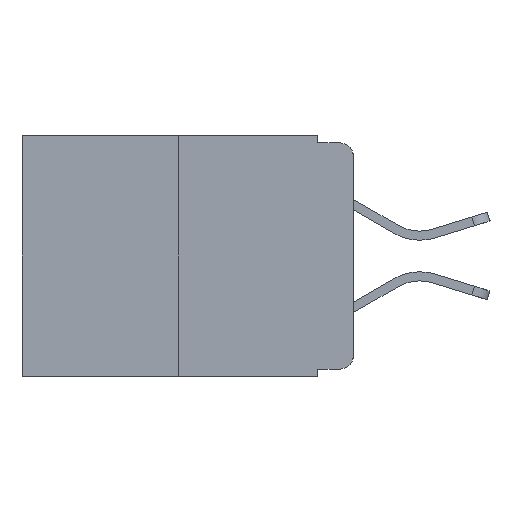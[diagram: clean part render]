
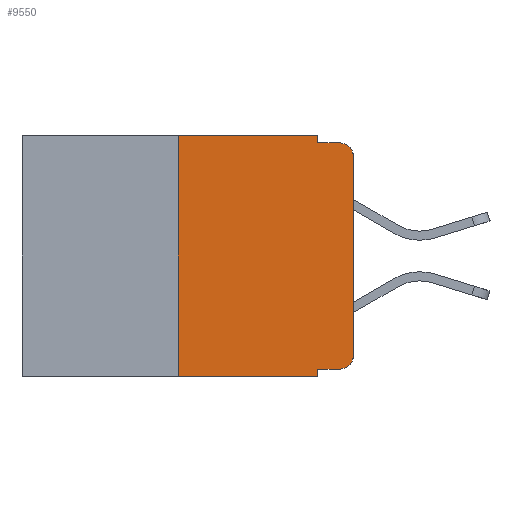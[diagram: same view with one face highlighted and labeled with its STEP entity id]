
A CAD part, left-side view. The second image highlights one B-rep face of the part: STEP entity #9550.
In plain terms, the highlighted planar face has unit normal (-1, 0, 0).
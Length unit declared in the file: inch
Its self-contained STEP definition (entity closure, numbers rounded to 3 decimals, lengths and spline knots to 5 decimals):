
#59 = VECTOR ( 'NONE', #10733, 39.37008 ) ;
#154 = AXIS2_PLACEMENT_3D ( 'NONE', #11828, #5738, #11857 ) ;
#215 = ORIENTED_EDGE ( 'NONE', *, *, #3787, .F. ) ;
#564 = ORIENTED_EDGE ( 'NONE', *, *, #3945, .F. ) ;
#913 = CARTESIAN_POINT ( 'NONE',  ( 0., 0.473, 0. ) ) ;
#932 = CIRCLE ( 'NONE', #11629, 0.02 ) ;
#991 = ORIENTED_EDGE ( 'NONE', *, *, #3729, .T. ) ;
#1109 = VECTOR ( 'NONE', #10642, 39.37008 ) ;
#1373 = VERTEX_POINT ( 'NONE', #12128 ) ;
#1569 = VERTEX_POINT ( 'NONE', #6097 ) ;
#2163 = CARTESIAN_POINT ( 'NONE',  ( 0., 0.25, 0. ) ) ;
#2320 = ORIENTED_EDGE ( 'NONE', *, *, #3783, .T. ) ;
#2646 = ORIENTED_EDGE ( 'NONE', *, *, #3926, .T. ) ;
#3071 = VECTOR ( 'NONE', #6864, 39.37008 ) ;
#3140 = CARTESIAN_POINT ( 'NONE',  ( 0., 0.051, -0.343 ) ) ;
#3144 = VECTOR ( 'NONE', #8566, 39.37008 ) ;
#3314 = LINE ( 'NONE', #11605, #8231 ) ;
#3404 = DIRECTION ( 'NONE',  ( 0., -1., 0. ) ) ;
#3415 = LINE ( 'NONE', #913, #3071 ) ;
#3512 = FACE_OUTER_BOUND ( 'NONE', #10584, .T. ) ;
#3526 = ORIENTED_EDGE ( 'NONE', *, *, #3968, .T. ) ;
#3618 = LINE ( 'NONE', #11308, #10533 ) ;
#3729 = EDGE_CURVE ( 'NONE', #11973, #4714, #6537, .T. ) ;
#3783 = EDGE_CURVE ( 'NONE', #4714, #11696, #932, .T. ) ;
#3787 = EDGE_CURVE ( 'NONE', #5689, #11696, #5661, .T. ) ;
#3902 = CARTESIAN_POINT ( 'NONE',  ( 0., 0.051, 0. ) ) ;
#3912 = EDGE_CURVE ( 'NONE', #5344, #5689, #11057, .T. ) ;
#3914 = EDGE_CURVE ( 'NONE', #1569, #8278, #3940, .T. ) ;
#3926 = EDGE_CURVE ( 'NONE', #4440, #1373, #3618, .T. ) ;
#3940 = LINE ( 'NONE', #11932, #6104 ) ;
#3945 = EDGE_CURVE ( 'NONE', #4440, #7474, #3314, .T. ) ;
#3968 = EDGE_CURVE ( 'NONE', #1373, #11973, #7937, .T. ) ;
#4101 = VECTOR ( 'NONE', #5047, 39.37008 ) ;
#4348 = DIRECTION ( 'NONE',  ( 0., 0., -1. ) ) ;
#4440 = VERTEX_POINT ( 'NONE', #9149 ) ;
#4520 = CARTESIAN_POINT ( 'NONE',  ( 0., 0.473, -0.343 ) ) ;
#4714 = VERTEX_POINT ( 'NONE', #7697 ) ;
#4834 = PLANE ( 'NONE',  #154 ) ;
#5047 = DIRECTION ( 'NONE',  ( 0., 0., 1. ) ) ;
#5276 = LINE ( 'NONE', #4520, #59 ) ;
#5344 = VERTEX_POINT ( 'NONE', #3902 ) ;
#5661 = LINE ( 'NONE', #6127, #3144 ) ;
#5689 = VERTEX_POINT ( 'NONE', #9738 ) ;
#5738 = DIRECTION ( 'NONE',  ( 1., 0., 0. ) ) ;
#5797 = CARTESIAN_POINT ( 'NONE',  ( 0., 0.02, -0.01 ) ) ;
#6089 = DIRECTION ( 'NONE',  ( 0., 0., 1. ) ) ;
#6097 = CARTESIAN_POINT ( 'NONE',  ( 0., 0.25, -0.343 ) ) ;
#6104 = VECTOR ( 'NONE', #6089, 39.37008 ) ;
#6127 = CARTESIAN_POINT ( 'NONE',  ( 0., 0.051, -0.01 ) ) ;
#6133 = AXIS2_PLACEMENT_3D ( 'NONE', #10855, #11902, #8687 ) ;
#6362 = ORIENTED_EDGE ( 'NONE', *, *, #3912, .F. ) ;
#6537 = LINE ( 'NONE', #10196, #4101 ) ;
#6864 = DIRECTION ( 'NONE',  ( 0., -1., 0. ) ) ;
#7067 = ORIENTED_EDGE ( 'NONE', *, *, #7230, .F. ) ;
#7163 = ORIENTED_EDGE ( 'NONE', *, *, #3914, .F. ) ;
#7208 = DIRECTION ( 'NONE',  ( -1., 0., 0. ) ) ;
#7230 = EDGE_CURVE ( 'NONE', #8278, #5344, #3415, .T. ) ;
#7474 = VERTEX_POINT ( 'NONE', #3140 ) ;
#7697 = CARTESIAN_POINT ( 'NONE',  ( 0., 0., -0.03 ) ) ;
#7937 = CIRCLE ( 'NONE', #6133, 0.02 ) ;
#7986 = CARTESIAN_POINT ( 'NONE',  ( 0., 0., -0.313 ) ) ;
#8211 = ORIENTED_EDGE ( 'NONE', *, *, #12188, .T. ) ;
#8231 = VECTOR ( 'NONE', #4348, 39.37008 ) ;
#8278 = VERTEX_POINT ( 'NONE', #2163 ) ;
#8566 = DIRECTION ( 'NONE',  ( 0., -1., 0. ) ) ;
#8687 = DIRECTION ( 'NONE',  ( 0., 0., -1. ) ) ;
#9149 = CARTESIAN_POINT ( 'NONE',  ( 0., 0.051, -0.333 ) ) ;
#9550 = ADVANCED_FACE ( 'NONE', ( #3512 ), #4834, .F. ) ;
#9738 = CARTESIAN_POINT ( 'NONE',  ( 0., 0.051, -0.01 ) ) ;
#10196 = CARTESIAN_POINT ( 'NONE',  ( 0., 0., 0. ) ) ;
#10299 = CARTESIAN_POINT ( 'NONE',  ( 0., 0.02, -0.03 ) ) ;
#10533 = VECTOR ( 'NONE', #3404, 39.37008 ) ;
#10584 = EDGE_LOOP ( 'NONE', ( #991, #2320, #215, #6362, #7067, #7163, #8211, #564, #2646, #3526 ) ) ;
#10590 = DIRECTION ( 'NONE',  ( 0., 0., -1. ) ) ;
#10642 = DIRECTION ( 'NONE',  ( 0., 0., -1. ) ) ;
#10733 = DIRECTION ( 'NONE',  ( 0., -1., 0. ) ) ;
#10855 = CARTESIAN_POINT ( 'NONE',  ( 0., 0.02, -0.313 ) ) ;
#11057 = LINE ( 'NONE', #12155, #1109 ) ;
#11308 = CARTESIAN_POINT ( 'NONE',  ( 0., 0.051, -0.333 ) ) ;
#11605 = CARTESIAN_POINT ( 'NONE',  ( 0., 0.051, 0. ) ) ;
#11629 = AXIS2_PLACEMENT_3D ( 'NONE', #10299, #7208, #10590 ) ;
#11696 = VERTEX_POINT ( 'NONE', #5797 ) ;
#11828 = CARTESIAN_POINT ( 'NONE',  ( 0., 0.473, 0. ) ) ;
#11857 = DIRECTION ( 'NONE',  ( 0., 0., -1. ) ) ;
#11902 = DIRECTION ( 'NONE',  ( -1., 0., 0. ) ) ;
#11932 = CARTESIAN_POINT ( 'NONE',  ( 0., 0.25, 0. ) ) ;
#11973 = VERTEX_POINT ( 'NONE', #7986 ) ;
#12128 = CARTESIAN_POINT ( 'NONE',  ( 0., 0.02, -0.333 ) ) ;
#12155 = CARTESIAN_POINT ( 'NONE',  ( 0., 0.051, 0. ) ) ;
#12188 = EDGE_CURVE ( 'NONE', #1569, #7474, #5276, .T. ) ;
